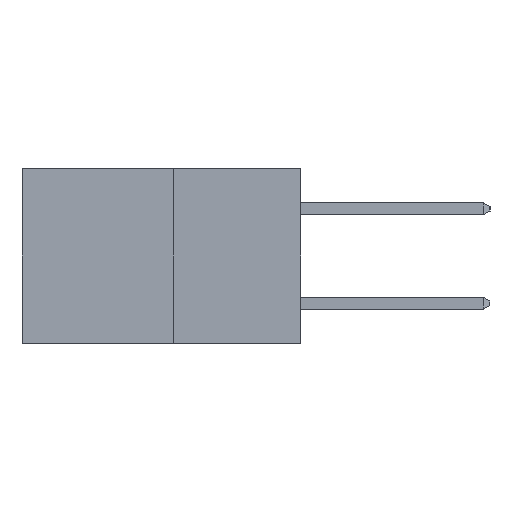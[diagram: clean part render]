
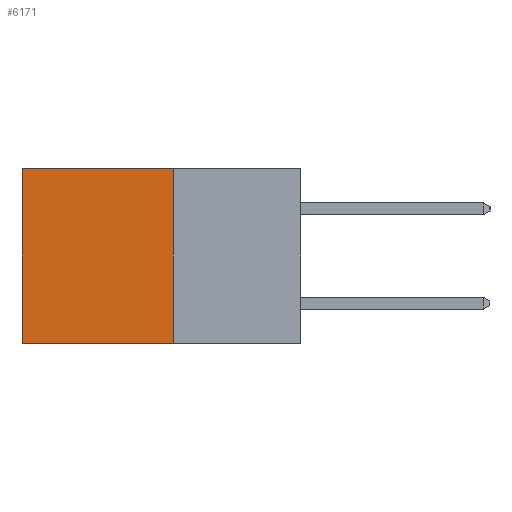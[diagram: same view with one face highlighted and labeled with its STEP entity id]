
A CAD part, left-side view. The second image highlights one B-rep face of the part: STEP entity #6171.
In plain terms, the highlighted planar face has unit normal (-1, 0, 0).
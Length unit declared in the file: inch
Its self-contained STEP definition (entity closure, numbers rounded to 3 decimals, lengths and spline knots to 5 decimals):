
#399 = LINE ( 'NONE', #7954, #2905 ) ;
#782 = EDGE_CURVE ( 'NONE', #10303, #10710, #2954, .T. ) ;
#1099 = EDGE_CURVE ( 'NONE', #10303, #7775, #9899, .T. ) ;
#1161 = CARTESIAN_POINT ( 'NONE',  ( 0.277, 0.27, -0.37 ) ) ;
#2388 = CARTESIAN_POINT ( 'NONE',  ( 0.277, 0.27, 0. ) ) ;
#2905 = VECTOR ( 'NONE', #6811, 39.37008 ) ;
#2954 = LINE ( 'NONE', #9779, #8282 ) ;
#3117 = CARTESIAN_POINT ( 'NONE',  ( 0.277, 0.59, 0. ) ) ;
#3840 = DIRECTION ( 'NONE',  ( 0., 0., -1. ) ) ;
#3911 = EDGE_CURVE ( 'NONE', #10710, #10623, #13506, .T. ) ;
#3920 = PLANE ( 'NONE',  #4475 ) ;
#4256 = ORIENTED_EDGE ( 'NONE', *, *, #782, .T. ) ;
#4475 = AXIS2_PLACEMENT_3D ( 'NONE', #1161, #5730, #5532 ) ;
#4552 = ORIENTED_EDGE ( 'NONE', *, *, #1099, .F. ) ;
#5072 = CARTESIAN_POINT ( 'NONE',  ( 0.277, 0.59, -0.37 ) ) ;
#5532 = DIRECTION ( 'NONE',  ( 0., 0., -1. ) ) ;
#5730 = DIRECTION ( 'NONE',  ( 1., 0., 0. ) ) ;
#5739 = EDGE_CURVE ( 'NONE', #7775, #10623, #399, .T. ) ;
#6171 = ADVANCED_FACE ( 'NONE', ( #6419 ), #3920, .F. ) ;
#6401 = CARTESIAN_POINT ( 'NONE',  ( 0.277, 0.27, -0.37 ) ) ;
#6419 = FACE_OUTER_BOUND ( 'NONE', #8536, .T. ) ;
#6807 = ORIENTED_EDGE ( 'NONE', *, *, #3911, .T. ) ;
#6811 = DIRECTION ( 'NONE',  ( 0., 1., 0. ) ) ;
#7220 = CARTESIAN_POINT ( 'NONE',  ( 0.277, 0.27, -0.37 ) ) ;
#7270 = DIRECTION ( 'NONE',  ( 0., 1., 0. ) ) ;
#7775 = VERTEX_POINT ( 'NONE', #6401 ) ;
#7794 = ORIENTED_EDGE ( 'NONE', *, *, #5739, .F. ) ;
#7954 = CARTESIAN_POINT ( 'NONE',  ( 0.277, 0.27, -0.37 ) ) ;
#8282 = VECTOR ( 'NONE', #7270, 39.37008 ) ;
#8536 = EDGE_LOOP ( 'NONE', ( #6807, #7794, #4552, #4256 ) ) ;
#8730 = VECTOR ( 'NONE', #10731, 39.37008 ) ;
#9564 = VECTOR ( 'NONE', #3840, 39.37008 ) ;
#9737 = CARTESIAN_POINT ( 'NONE',  ( 0.277, 0.59, -0.37 ) ) ;
#9779 = CARTESIAN_POINT ( 'NONE',  ( 0.277, 0.27, 0. ) ) ;
#9899 = LINE ( 'NONE', #7220, #9564 ) ;
#10303 = VERTEX_POINT ( 'NONE', #2388 ) ;
#10623 = VERTEX_POINT ( 'NONE', #5072 ) ;
#10710 = VERTEX_POINT ( 'NONE', #3117 ) ;
#10731 = DIRECTION ( 'NONE',  ( 0., 0., -1. ) ) ;
#13506 = LINE ( 'NONE', #9737, #8730 ) ;
